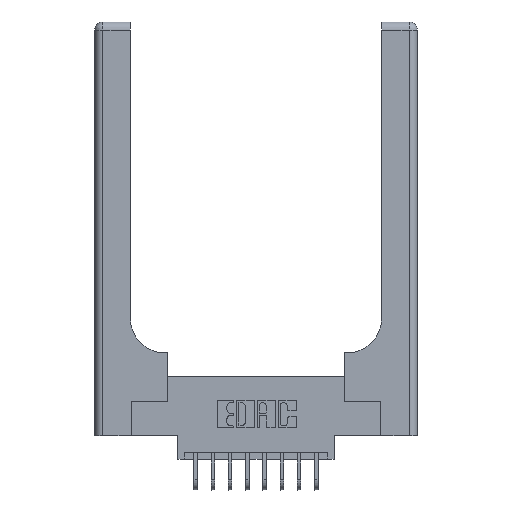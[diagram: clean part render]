
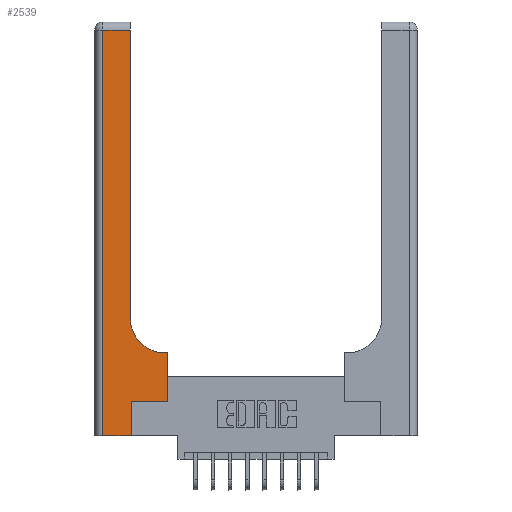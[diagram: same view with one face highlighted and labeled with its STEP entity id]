
A CAD part, top view. The second image highlights one B-rep face of the part: STEP entity #2539.
In plain terms, the highlighted planar face has unit normal (0, 0, 1).
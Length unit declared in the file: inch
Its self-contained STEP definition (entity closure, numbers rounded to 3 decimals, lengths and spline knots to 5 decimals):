
#30 = DIRECTION ( 'NONE',  ( 1., 0., 0. ) ) ;
#135 = CARTESIAN_POINT ( 'NONE',  ( 0.265, 0.25, 0.37 ) ) ;
#207 = EDGE_CURVE ( 'NONE', #17307, #16212, #13978, .T. ) ;
#373 = VECTOR ( 'NONE', #1737, 39.37008 ) ;
#447 = DIRECTION ( 'NONE',  ( -1., 0., 0. ) ) ;
#723 = AXIS2_PLACEMENT_3D ( 'NONE', #9417, #10832, #14790 ) ;
#987 = CARTESIAN_POINT ( 'NONE',  ( 0.26, 0.6, 0.37 ) ) ;
#1028 = VERTEX_POINT ( 'NONE', #5246 ) ;
#1048 = VECTOR ( 'NONE', #3737, 39.37008 ) ;
#1561 = VERTEX_POINT ( 'NONE', #5866 ) ;
#1737 = DIRECTION ( 'NONE',  ( 0., 1., 0. ) ) ;
#1763 = CARTESIAN_POINT ( 'NONE',  ( 0.265, 0., 0.37 ) ) ;
#1896 = LINE ( 'NONE', #9712, #13687 ) ;
#2074 = VECTOR ( 'NONE', #447, 39.37008 ) ;
#2539 = ADVANCED_FACE ( 'NONE', ( #15920 ), #17315, .F. ) ;
#2554 = AXIS2_PLACEMENT_3D ( 'NONE', #14682, #3800, #7733 ) ;
#2846 = ORIENTED_EDGE ( 'NONE', *, *, #9898, .T. ) ;
#2999 = LINE ( 'NONE', #1763, #12132 ) ;
#3102 = VECTOR ( 'NONE', #30, 39.37008 ) ;
#3274 = EDGE_LOOP ( 'NONE', ( #15667, #4822, #7707, #9335, #2846, #15432, #9746, #9359, #13667 ) ) ;
#3737 = DIRECTION ( 'NONE',  ( 0., -1., 0. ) ) ;
#3755 = VERTEX_POINT ( 'NONE', #10833 ) ;
#3800 = DIRECTION ( 'NONE',  ( 0., 0., -1. ) ) ;
#3945 = EDGE_CURVE ( 'NONE', #10321, #16000, #13027, .T. ) ;
#4659 = CARTESIAN_POINT ( 'NONE',  ( 0., 2.94, 0.37 ) ) ;
#4822 = ORIENTED_EDGE ( 'NONE', *, *, #207, .T. ) ;
#5246 = CARTESIAN_POINT ( 'NONE',  ( 0.528, 0.25, 0.37 ) ) ;
#5652 = DIRECTION ( 'NONE',  ( 0., 1., 0. ) ) ;
#5866 = CARTESIAN_POINT ( 'NONE',  ( 0.265, 0.25, 0.37 ) ) ;
#5944 = EDGE_CURVE ( 'NONE', #1028, #10321, #16306, .T. ) ;
#6619 = CARTESIAN_POINT ( 'NONE',  ( 0.528, 0.6, 0.37 ) ) ;
#6893 = DIRECTION ( 'NONE',  ( 1., 0., 0. ) ) ;
#7602 = EDGE_CURVE ( 'NONE', #16176, #16588, #14784, .T. ) ;
#7707 = ORIENTED_EDGE ( 'NONE', *, *, #14338, .T. ) ;
#7733 = DIRECTION ( 'NONE',  ( 1., 0., 0. ) ) ;
#8172 = EDGE_CURVE ( 'NONE', #16000, #3755, #13487, .T. ) ;
#8894 = CARTESIAN_POINT ( 'NONE',  ( 0.06, 3., 0.37 ) ) ;
#9204 = EDGE_CURVE ( 'NONE', #1561, #1028, #10770, .T. ) ;
#9335 = ORIENTED_EDGE ( 'NONE', *, *, #7602, .T. ) ;
#9359 = ORIENTED_EDGE ( 'NONE', *, *, #3945, .T. ) ;
#9417 = CARTESIAN_POINT ( 'NONE',  ( 0., 3., 0.37 ) ) ;
#9712 = CARTESIAN_POINT ( 'NONE',  ( 0.26, 3., 0.37 ) ) ;
#9746 = ORIENTED_EDGE ( 'NONE', *, *, #5944, .T. ) ;
#9811 = CARTESIAN_POINT ( 'NONE',  ( 0.528, 0.25, 0.37 ) ) ;
#9825 = CARTESIAN_POINT ( 'NONE',  ( 0.06, 0., 0.37 ) ) ;
#9898 = EDGE_CURVE ( 'NONE', #16588, #1561, #2999, .T. ) ;
#10298 = DIRECTION ( 'NONE',  ( -1., 0., 0. ) ) ;
#10321 = VERTEX_POINT ( 'NONE', #6619 ) ;
#10707 = VECTOR ( 'NONE', #6893, 39.37008 ) ;
#10770 = LINE ( 'NONE', #135, #10707 ) ;
#10832 = DIRECTION ( 'NONE',  ( 0., 0., -1. ) ) ;
#10833 = CARTESIAN_POINT ( 'NONE',  ( 0.26, 0.85, 0.37 ) ) ;
#12132 = VECTOR ( 'NONE', #14947, 39.37008 ) ;
#13027 = LINE ( 'NONE', #987, #16258 ) ;
#13123 = LINE ( 'NONE', #8894, #1048 ) ;
#13487 = CIRCLE ( 'NONE', #2554, 0.25 ) ;
#13667 = ORIENTED_EDGE ( 'NONE', *, *, #8172, .T. ) ;
#13687 = VECTOR ( 'NONE', #5652, 39.37008 ) ;
#13875 = CARTESIAN_POINT ( 'NONE',  ( 0.06, 2.94, 0.37 ) ) ;
#13941 = CARTESIAN_POINT ( 'NONE',  ( 0.265, 0., 0.37 ) ) ;
#13978 = LINE ( 'NONE', #4659, #2074 ) ;
#14338 = EDGE_CURVE ( 'NONE', #16212, #16176, #13123, .T. ) ;
#14682 = CARTESIAN_POINT ( 'NONE',  ( 0.51, 0.85, 0.37 ) ) ;
#14685 = CARTESIAN_POINT ( 'NONE',  ( 0.51, 0.6, 0.37 ) ) ;
#14784 = LINE ( 'NONE', #15747, #3102 ) ;
#14790 = DIRECTION ( 'NONE',  ( -1., 0., 0. ) ) ;
#14947 = DIRECTION ( 'NONE',  ( 0., 1., 0. ) ) ;
#15122 = CARTESIAN_POINT ( 'NONE',  ( 0.26, 2.94, 0.37 ) ) ;
#15296 = EDGE_CURVE ( 'NONE', #3755, #17307, #1896, .T. ) ;
#15432 = ORIENTED_EDGE ( 'NONE', *, *, #9204, .T. ) ;
#15667 = ORIENTED_EDGE ( 'NONE', *, *, #15296, .T. ) ;
#15747 = CARTESIAN_POINT ( 'NONE',  ( 0., 0., 0.37 ) ) ;
#15920 = FACE_OUTER_BOUND ( 'NONE', #3274, .T. ) ;
#16000 = VERTEX_POINT ( 'NONE', #14685 ) ;
#16176 = VERTEX_POINT ( 'NONE', #9825 ) ;
#16212 = VERTEX_POINT ( 'NONE', #13875 ) ;
#16258 = VECTOR ( 'NONE', #10298, 39.37008 ) ;
#16306 = LINE ( 'NONE', #9811, #373 ) ;
#16588 = VERTEX_POINT ( 'NONE', #13941 ) ;
#17307 = VERTEX_POINT ( 'NONE', #15122 ) ;
#17315 = PLANE ( 'NONE',  #723 ) ;
